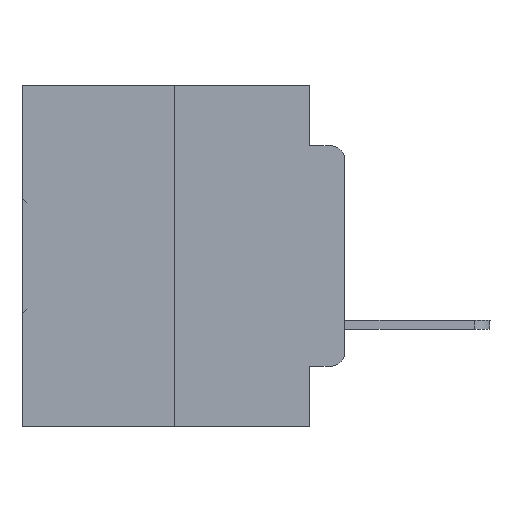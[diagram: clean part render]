
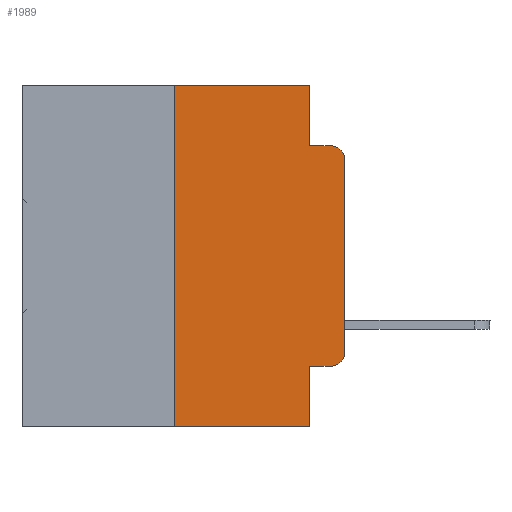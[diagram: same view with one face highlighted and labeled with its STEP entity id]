
A CAD part, left-side view. The second image highlights one B-rep face of the part: STEP entity #1989.
In plain terms, the highlighted planar face has unit normal (-1, 0, 0).
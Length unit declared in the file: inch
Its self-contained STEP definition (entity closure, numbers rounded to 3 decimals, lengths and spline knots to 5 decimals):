
#414 = DIRECTION ( 'NONE',  ( 0., 0., -1. ) ) ;
#724 = LINE ( 'NONE', #8958, #12902 ) ;
#1964 = EDGE_CURVE ( 'NONE', #5221, #33166, #30600, .T. ) ;
#1971 = LINE ( 'NONE', #25735, #21428 ) ;
#1989 = ADVANCED_FACE ( 'NONE', ( #23689 ), #7989, .F. ) ;
#2639 = CARTESIAN_POINT ( 'NONE',  ( 0., 0.473, 0. ) ) ;
#3395 = DIRECTION ( 'NONE',  ( 0., 0., -1. ) ) ;
#3504 = VECTOR ( 'NONE', #26591, 39.37008 ) ;
#3755 = CIRCLE ( 'NONE', #30896, 0.02 ) ;
#3816 = VERTEX_POINT ( 'NONE', #11131 ) ;
#3979 = CARTESIAN_POINT ( 'NONE',  ( 0., 0.473, 0. ) ) ;
#5221 = VERTEX_POINT ( 'NONE', #33483 ) ;
#5628 = VERTEX_POINT ( 'NONE', #18611 ) ;
#6221 = CARTESIAN_POINT ( 'NONE',  ( 0., 0.051, -0.0885 ) ) ;
#6235 = CARTESIAN_POINT ( 'NONE',  ( 0., 0.051, -0.5 ) ) ;
#6583 = DIRECTION ( 'NONE',  ( 0., -1., 0. ) ) ;
#6606 = ORIENTED_EDGE ( 'NONE', *, *, #32674, .F. ) ;
#7045 = ORIENTED_EDGE ( 'NONE', *, *, #30157, .F. ) ;
#7377 = EDGE_CURVE ( 'NONE', #11011, #3816, #3755, .T. ) ;
#7420 = VERTEX_POINT ( 'NONE', #6235 ) ;
#7735 = EDGE_CURVE ( 'NONE', #5628, #11011, #1971, .T. ) ;
#7974 = DIRECTION ( 'NONE',  ( 0., -1., 0. ) ) ;
#7989 = PLANE ( 'NONE',  #33718 ) ;
#8320 = EDGE_CURVE ( 'NONE', #33166, #5628, #26507, .T. ) ;
#8504 = DIRECTION ( 'NONE',  ( -1., 0., 0. ) ) ;
#8524 = ORIENTED_EDGE ( 'NONE', *, *, #7377, .T. ) ;
#8958 = CARTESIAN_POINT ( 'NONE',  ( 0., 0.051, 0. ) ) ;
#8971 = VECTOR ( 'NONE', #7974, 39.37008 ) ;
#9550 = CARTESIAN_POINT ( 'NONE',  ( 0., 0.051, 0. ) ) ;
#9780 = CARTESIAN_POINT ( 'NONE',  ( 0., 0.051, 0. ) ) ;
#9984 = ORIENTED_EDGE ( 'NONE', *, *, #26352, .F. ) ;
#10032 = CARTESIAN_POINT ( 'NONE',  ( 0., 0.25, 0. ) ) ;
#10059 = DIRECTION ( 'NONE',  ( 0., 0., 1. ) ) ;
#10601 = ORIENTED_EDGE ( 'NONE', *, *, #31190, .F. ) ;
#10626 = CARTESIAN_POINT ( 'NONE',  ( 0., 0., -0.1085 ) ) ;
#10643 = CARTESIAN_POINT ( 'NONE',  ( 0., 0.02, -0.3915 ) ) ;
#10797 = LINE ( 'NONE', #14337, #3504 ) ;
#11011 = VERTEX_POINT ( 'NONE', #10626 ) ;
#11088 = DIRECTION ( 'NONE',  ( 0., -1., 0. ) ) ;
#11131 = CARTESIAN_POINT ( 'NONE',  ( 0., 0.02, -0.0885 ) ) ;
#12902 = VECTOR ( 'NONE', #3395, 39.37008 ) ;
#13763 = ORIENTED_EDGE ( 'NONE', *, *, #7735, .T. ) ;
#13788 = VERTEX_POINT ( 'NONE', #10032 ) ;
#14005 = EDGE_CURVE ( 'NONE', #5221, #7420, #33035, .T. ) ;
#14337 = CARTESIAN_POINT ( 'NONE',  ( 0., 0.051, -0.0885 ) ) ;
#15365 = DIRECTION ( 'NONE',  ( 1., 0., 0. ) ) ;
#15822 = EDGE_CURVE ( 'NONE', #19288, #7420, #27894, .T. ) ;
#17869 = DIRECTION ( 'NONE',  ( 0., 0., 1. ) ) ;
#18541 = CARTESIAN_POINT ( 'NONE',  ( 0., 0.02, -0.1085 ) ) ;
#18611 = CARTESIAN_POINT ( 'NONE',  ( 0., 0., -0.3915 ) ) ;
#19288 = VERTEX_POINT ( 'NONE', #19713 ) ;
#19591 = AXIS2_PLACEMENT_3D ( 'NONE', #10643, #20839, #28918 ) ;
#19713 = CARTESIAN_POINT ( 'NONE',  ( 0., 0.25, -0.5 ) ) ;
#20065 = ORIENTED_EDGE ( 'NONE', *, *, #8320, .T. ) ;
#20595 = ORIENTED_EDGE ( 'NONE', *, *, #14005, .F. ) ;
#20735 = CARTESIAN_POINT ( 'NONE',  ( 0., 0.25, 0. ) ) ;
#20839 = DIRECTION ( 'NONE',  ( -1., 0., 0. ) ) ;
#20947 = VECTOR ( 'NONE', #11088, 39.37008 ) ;
#21138 = VECTOR ( 'NONE', #6583, 39.37008 ) ;
#21428 = VECTOR ( 'NONE', #10059, 39.37008 ) ;
#22438 = CARTESIAN_POINT ( 'NONE',  ( 0., 0.02, -0.4115 ) ) ;
#23502 = CARTESIAN_POINT ( 'NONE',  ( 0., 0.051, -0.4115 ) ) ;
#23689 = FACE_OUTER_BOUND ( 'NONE', #25602, .T. ) ;
#24082 = VECTOR ( 'NONE', #33801, 39.37008 ) ;
#24361 = ORIENTED_EDGE ( 'NONE', *, *, #1964, .T. ) ;
#24551 = ORIENTED_EDGE ( 'NONE', *, *, #15822, .T. ) ;
#25602 = EDGE_LOOP ( 'NONE', ( #13763, #8524, #9984, #10601, #7045, #6606, #24551, #20595, #24361, #20065 ) ) ;
#25735 = CARTESIAN_POINT ( 'NONE',  ( 0., 0., 0. ) ) ;
#26352 = EDGE_CURVE ( 'NONE', #30659, #3816, #10797, .T. ) ;
#26507 = CIRCLE ( 'NONE', #19591, 0.02 ) ;
#26517 = VERTEX_POINT ( 'NONE', #9550 ) ;
#26591 = DIRECTION ( 'NONE',  ( 0., -1., 0. ) ) ;
#27894 = LINE ( 'NONE', #29696, #20947 ) ;
#28918 = DIRECTION ( 'NONE',  ( 0., 0., -1. ) ) ;
#29696 = CARTESIAN_POINT ( 'NONE',  ( 0., 0.473, -0.5 ) ) ;
#30157 = EDGE_CURVE ( 'NONE', #13788, #26517, #32523, .T. ) ;
#30600 = LINE ( 'NONE', #23502, #8971 ) ;
#30659 = VERTEX_POINT ( 'NONE', #6221 ) ;
#30698 = VECTOR ( 'NONE', #17869, 39.37008 ) ;
#30896 = AXIS2_PLACEMENT_3D ( 'NONE', #18541, #8504, #414 ) ;
#31190 = EDGE_CURVE ( 'NONE', #26517, #30659, #724, .T. ) ;
#31440 = DIRECTION ( 'NONE',  ( 0., 0., -1. ) ) ;
#31892 = LINE ( 'NONE', #20735, #30698 ) ;
#32523 = LINE ( 'NONE', #3979, #21138 ) ;
#32674 = EDGE_CURVE ( 'NONE', #19288, #13788, #31892, .T. ) ;
#33035 = LINE ( 'NONE', #9780, #24082 ) ;
#33166 = VERTEX_POINT ( 'NONE', #22438 ) ;
#33483 = CARTESIAN_POINT ( 'NONE',  ( 0., 0.051, -0.4115 ) ) ;
#33718 = AXIS2_PLACEMENT_3D ( 'NONE', #2639, #15365, #31440 ) ;
#33801 = DIRECTION ( 'NONE',  ( 0., 0., -1. ) ) ;
